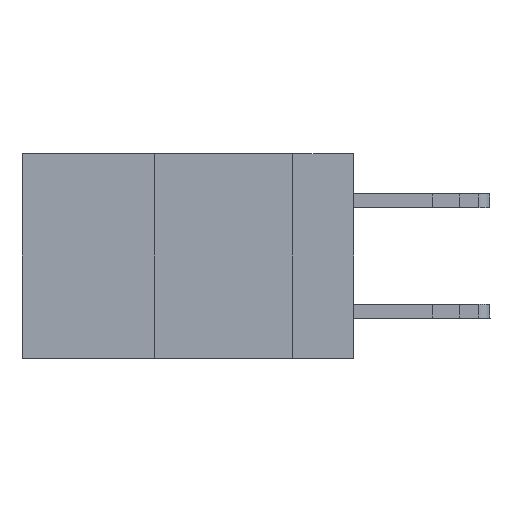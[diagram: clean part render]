
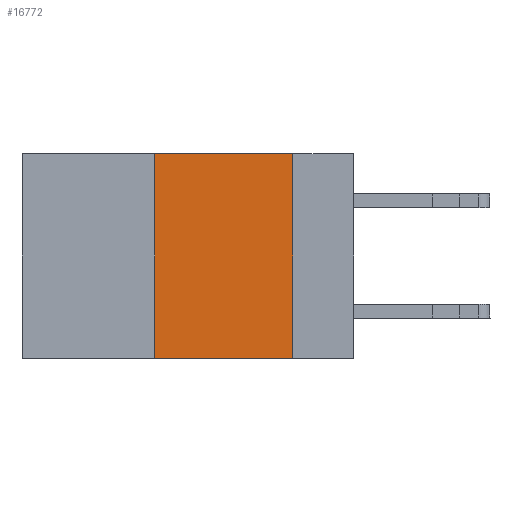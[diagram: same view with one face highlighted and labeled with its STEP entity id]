
A CAD part, left-side view. The second image highlights one B-rep face of the part: STEP entity #16772.
In plain terms, the highlighted planar face has unit normal (-1, 0, 0).
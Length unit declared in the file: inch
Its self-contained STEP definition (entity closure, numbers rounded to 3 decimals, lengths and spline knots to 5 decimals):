
#763 = LINE ( 'NONE', #12829, #6666 ) ;
#958 = VERTEX_POINT ( 'NONE', #2100 ) ;
#985 = PLANE ( 'NONE',  #11934 ) ;
#2041 = DIRECTION ( 'NONE',  ( 0., -1., 0. ) ) ;
#2100 = CARTESIAN_POINT ( 'NONE',  ( 0., 0.36, -0.37 ) ) ;
#2157 = VECTOR ( 'NONE', #9501, 39.37008 ) ;
#4639 = DIRECTION ( 'NONE',  ( 0., 0., -1. ) ) ;
#5609 = CARTESIAN_POINT ( 'NONE',  ( 0., 0.36, 0. ) ) ;
#6666 = VECTOR ( 'NONE', #2041, 39.37008 ) ;
#7750 = CARTESIAN_POINT ( 'NONE',  ( 0., 0.11, 0. ) ) ;
#8636 = ORIENTED_EDGE ( 'NONE', *, *, #22709, .F. ) ;
#8872 = VERTEX_POINT ( 'NONE', #20825 ) ;
#9501 = DIRECTION ( 'NONE',  ( 0., 0., -1. ) ) ;
#9623 = VERTEX_POINT ( 'NONE', #15977 ) ;
#9710 = FACE_OUTER_BOUND ( 'NONE', #18142, .T. ) ;
#9913 = DIRECTION ( 'NONE',  ( 0., 0., 1. ) ) ;
#10960 = ORIENTED_EDGE ( 'NONE', *, *, #22559, .F. ) ;
#11934 = AXIS2_PLACEMENT_3D ( 'NONE', #13577, #15399, #4639 ) ;
#12231 = VERTEX_POINT ( 'NONE', #5609 ) ;
#12295 = LINE ( 'NONE', #7750, #2157 ) ;
#12829 = CARTESIAN_POINT ( 'NONE',  ( 0., 0.6, 0. ) ) ;
#12950 = ORIENTED_EDGE ( 'NONE', *, *, #20353, .F. ) ;
#13577 = CARTESIAN_POINT ( 'NONE',  ( 0., 0.6, 0. ) ) ;
#14022 = CARTESIAN_POINT ( 'NONE',  ( 0., 0.6, -0.37 ) ) ;
#14615 = LINE ( 'NONE', #14022, #18796 ) ;
#15399 = DIRECTION ( 'NONE',  ( 1., 0., 0. ) ) ;
#15638 = EDGE_CURVE ( 'NONE', #958, #9623, #14615, .T. ) ;
#15977 = CARTESIAN_POINT ( 'NONE',  ( 0., 0.11, -0.37 ) ) ;
#16081 = VECTOR ( 'NONE', #9913, 39.37008 ) ;
#16772 = ADVANCED_FACE ( 'NONE', ( #9710 ), #985, .F. ) ;
#17046 = ORIENTED_EDGE ( 'NONE', *, *, #15638, .T. ) ;
#18142 = EDGE_LOOP ( 'NONE', ( #8636, #10960, #12950, #17046 ) ) ;
#18796 = VECTOR ( 'NONE', #22689, 39.37008 ) ;
#20191 = LINE ( 'NONE', #20607, #16081 ) ;
#20353 = EDGE_CURVE ( 'NONE', #958, #12231, #20191, .T. ) ;
#20607 = CARTESIAN_POINT ( 'NONE',  ( 0., 0.36, 0. ) ) ;
#20825 = CARTESIAN_POINT ( 'NONE',  ( 0., 0.11, 0. ) ) ;
#22559 = EDGE_CURVE ( 'NONE', #12231, #8872, #763, .T. ) ;
#22689 = DIRECTION ( 'NONE',  ( 0., -1., 0. ) ) ;
#22709 = EDGE_CURVE ( 'NONE', #8872, #9623, #12295, .T. ) ;
